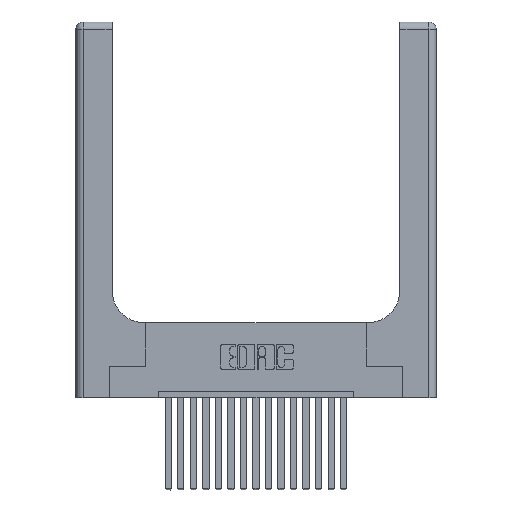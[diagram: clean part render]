
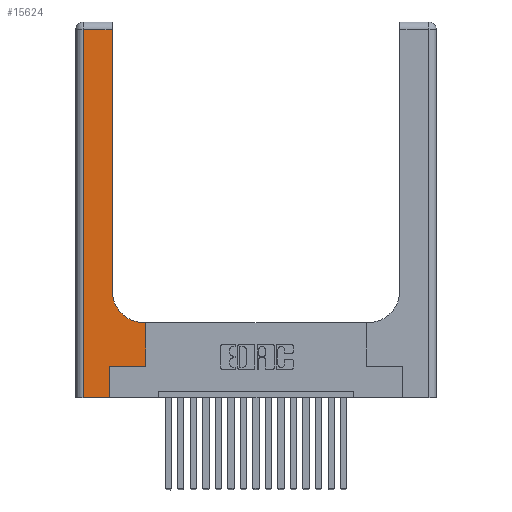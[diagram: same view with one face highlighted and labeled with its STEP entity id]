
A CAD part, top view. The second image highlights one B-rep face of the part: STEP entity #15624.
In plain terms, the highlighted planar face has unit normal (0, 0, 1).
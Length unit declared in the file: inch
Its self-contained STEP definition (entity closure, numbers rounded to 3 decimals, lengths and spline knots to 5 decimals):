
#219 = VERTEX_POINT ( 'NONE', #10189 ) ;
#384 = CARTESIAN_POINT ( 'NONE',  ( 0.269, 0.25, 0.37 ) ) ;
#653 = CARTESIAN_POINT ( 'NONE',  ( 0.06, 2.94, 0.37 ) ) ;
#677 = LINE ( 'NONE', #6064, #18473 ) ;
#690 = DIRECTION ( 'NONE',  ( 1., 0., 0. ) ) ;
#1246 = LINE ( 'NONE', #10771, #9936 ) ;
#1372 = CARTESIAN_POINT ( 'NONE',  ( 0.2915, 2.94, 0.37 ) ) ;
#1635 = EDGE_CURVE ( 'NONE', #4309, #10794, #16442, .T. ) ;
#1772 = VERTEX_POINT ( 'NONE', #12683 ) ;
#1923 = DIRECTION ( 'NONE',  ( 1., 0., 0. ) ) ;
#2004 = AXIS2_PLACEMENT_3D ( 'NONE', #9929, #12966, #690 ) ;
#2065 = VERTEX_POINT ( 'NONE', #1372 ) ;
#2411 = DIRECTION ( 'NONE',  ( 1., 0., 0. ) ) ;
#2427 = CARTESIAN_POINT ( 'NONE',  ( 0.2915, 3., 0.37 ) ) ;
#2770 = ORIENTED_EDGE ( 'NONE', *, *, #8661, .T. ) ;
#4050 = VERTEX_POINT ( 'NONE', #10506 ) ;
#4199 = EDGE_CURVE ( 'NONE', #2065, #14044, #16815, .T. ) ;
#4276 = DIRECTION ( 'NONE',  ( 0., 1., 0. ) ) ;
#4309 = VERTEX_POINT ( 'NONE', #6098 ) ;
#4971 = VECTOR ( 'NONE', #4276, 39.37008 ) ;
#5835 = LINE ( 'NONE', #19940, #8027 ) ;
#6064 = CARTESIAN_POINT ( 'NONE',  ( 0.2915, 0.6, 0.37 ) ) ;
#6098 = CARTESIAN_POINT ( 'NONE',  ( 0.269, 0., 0.37 ) ) ;
#6111 = EDGE_LOOP ( 'NONE', ( #12239, #9643, #11030, #9622, #11227, #17650, #2770, #7116, #19650 ) ) ;
#6185 = DIRECTION ( 'NONE',  ( 0., -1., 0. ) ) ;
#6308 = VECTOR ( 'NONE', #2411, 39.37008 ) ;
#6670 = DIRECTION ( 'NONE',  ( -1., 0., 0. ) ) ;
#7116 = ORIENTED_EDGE ( 'NONE', *, *, #17000, .T. ) ;
#7255 = LINE ( 'NONE', #9957, #6308 ) ;
#7623 = DIRECTION ( 'NONE',  ( -1., 0., 0. ) ) ;
#8027 = VECTOR ( 'NONE', #6185, 39.37008 ) ;
#8108 = EDGE_CURVE ( 'NONE', #10794, #1772, #19048, .T. ) ;
#8661 = EDGE_CURVE ( 'NONE', #1772, #4050, #1246, .T. ) ;
#8686 = VECTOR ( 'NONE', #17417, 39.37008 ) ;
#9622 = ORIENTED_EDGE ( 'NONE', *, *, #15659, .T. ) ;
#9643 = ORIENTED_EDGE ( 'NONE', *, *, #4199, .T. ) ;
#9929 = CARTESIAN_POINT ( 'NONE',  ( 0.5415, 0.85, 0.37 ) ) ;
#9936 = VECTOR ( 'NONE', #13949, 39.37008 ) ;
#9957 = CARTESIAN_POINT ( 'NONE',  ( 0., 0., 0.37 ) ) ;
#10189 = CARTESIAN_POINT ( 'NONE',  ( 0.06, 0., 0.37 ) ) ;
#10343 = VERTEX_POINT ( 'NONE', #17699 ) ;
#10423 = EDGE_CURVE ( 'NONE', #13364, #10343, #10821, .T. ) ;
#10506 = CARTESIAN_POINT ( 'NONE',  ( 0.5585, 0.6, 0.37 ) ) ;
#10771 = CARTESIAN_POINT ( 'NONE',  ( 0.5585, 0.25, 0.37 ) ) ;
#10794 = VERTEX_POINT ( 'NONE', #384 ) ;
#10821 = CIRCLE ( 'NONE', #2004, 0.25 ) ;
#11030 = ORIENTED_EDGE ( 'NONE', *, *, #12960, .T. ) ;
#11091 = FACE_OUTER_BOUND ( 'NONE', #6111, .T. ) ;
#11227 = ORIENTED_EDGE ( 'NONE', *, *, #1635, .T. ) ;
#11299 = CARTESIAN_POINT ( 'NONE',  ( 0., 3., 0.37 ) ) ;
#11916 = CARTESIAN_POINT ( 'NONE',  ( 0.269, 0., 0.37 ) ) ;
#12239 = ORIENTED_EDGE ( 'NONE', *, *, #16635, .T. ) ;
#12683 = CARTESIAN_POINT ( 'NONE',  ( 0.5585, 0.25, 0.37 ) ) ;
#12703 = CARTESIAN_POINT ( 'NONE',  ( 0., 2.94, 0.37 ) ) ;
#12798 = PLANE ( 'NONE',  #16357 ) ;
#12960 = EDGE_CURVE ( 'NONE', #14044, #219, #5835, .T. ) ;
#12966 = DIRECTION ( 'NONE',  ( 0., 0., -1. ) ) ;
#13364 = VERTEX_POINT ( 'NONE', #15554 ) ;
#13949 = DIRECTION ( 'NONE',  ( 0., 1., 0. ) ) ;
#14044 = VERTEX_POINT ( 'NONE', #653 ) ;
#14345 = DIRECTION ( 'NONE',  ( 0., 0., -1. ) ) ;
#15554 = CARTESIAN_POINT ( 'NONE',  ( 0.5415, 0.6, 0.37 ) ) ;
#15609 = VECTOR ( 'NONE', #17651, 39.37008 ) ;
#15624 = ADVANCED_FACE ( 'NONE', ( #11091 ), #12798, .F. ) ;
#15659 = EDGE_CURVE ( 'NONE', #219, #4309, #7255, .T. ) ;
#16357 = AXIS2_PLACEMENT_3D ( 'NONE', #11299, #14345, #6670 ) ;
#16394 = VECTOR ( 'NONE', #1923, 39.37008 ) ;
#16442 = LINE ( 'NONE', #11916, #4971 ) ;
#16635 = EDGE_CURVE ( 'NONE', #10343, #2065, #18238, .T. ) ;
#16815 = LINE ( 'NONE', #12703, #8686 ) ;
#17000 = EDGE_CURVE ( 'NONE', #4050, #13364, #677, .T. ) ;
#17417 = DIRECTION ( 'NONE',  ( -1., 0., 0. ) ) ;
#17650 = ORIENTED_EDGE ( 'NONE', *, *, #8108, .T. ) ;
#17651 = DIRECTION ( 'NONE',  ( 0., 1., 0. ) ) ;
#17699 = CARTESIAN_POINT ( 'NONE',  ( 0.2915, 0.85, 0.37 ) ) ;
#18238 = LINE ( 'NONE', #2427, #15609 ) ;
#18473 = VECTOR ( 'NONE', #7623, 39.37008 ) ;
#19048 = LINE ( 'NONE', #19795, #16394 ) ;
#19650 = ORIENTED_EDGE ( 'NONE', *, *, #10423, .T. ) ;
#19795 = CARTESIAN_POINT ( 'NONE',  ( 0.269, 0.25, 0.37 ) ) ;
#19940 = CARTESIAN_POINT ( 'NONE',  ( 0.06, 3., 0.37 ) ) ;
